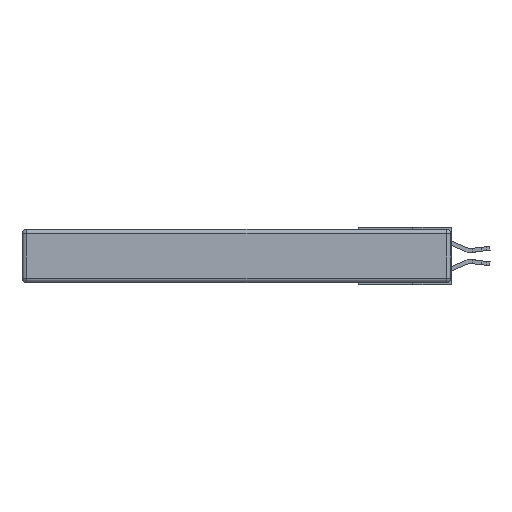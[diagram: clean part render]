
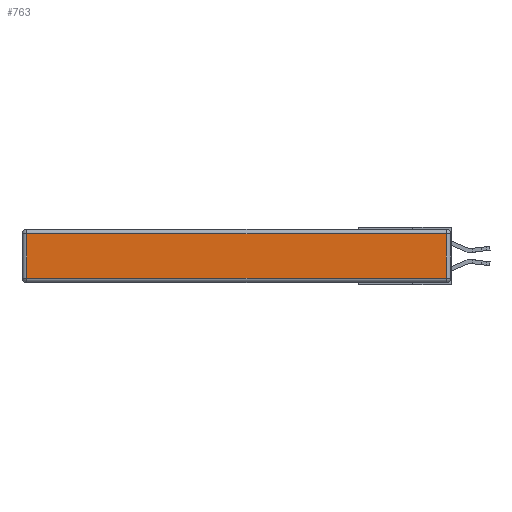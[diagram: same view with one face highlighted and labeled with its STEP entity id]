
A CAD part, left-side view. The second image highlights one B-rep face of the part: STEP entity #763.
In plain terms, the highlighted planar face has unit normal (-1, 0, 0).
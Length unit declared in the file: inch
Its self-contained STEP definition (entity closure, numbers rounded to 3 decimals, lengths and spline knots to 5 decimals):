
#692 = CARTESIAN_POINT ( 'NONE',  ( 0., 0., -0.343 ) ) ;
#763 = ADVANCED_FACE ( 'NONE', ( #19814 ), #5605, .T. ) ;
#936 = CARTESIAN_POINT ( 'NONE',  ( 0., 2.72, -0.313 ) ) ;
#1046 = CARTESIAN_POINT ( 'NONE',  ( 0., 0.03, -0.313 ) ) ;
#1474 = VECTOR ( 'NONE', #21287, 39.37008 ) ;
#1739 = LINE ( 'NONE', #4538, #1474 ) ;
#1753 = VECTOR ( 'NONE', #15206, 39.37008 ) ;
#2093 = EDGE_CURVE ( 'NONE', #3849, #6053, #13601, .T. ) ;
#2553 = EDGE_LOOP ( 'NONE', ( #14099, #6278, #18182, #12484 ) ) ;
#3849 = VERTEX_POINT ( 'NONE', #936 ) ;
#3950 = EDGE_CURVE ( 'NONE', #6053, #15411, #1739, .T. ) ;
#3998 = DIRECTION ( 'NONE',  ( 0., 0., 1. ) ) ;
#4538 = CARTESIAN_POINT ( 'NONE',  ( 0., 0.03, -0.343 ) ) ;
#5605 = PLANE ( 'NONE',  #11748 ) ;
#6053 = VERTEX_POINT ( 'NONE', #1046 ) ;
#6153 = CARTESIAN_POINT ( 'NONE',  ( 0., 0.03, -0.03 ) ) ;
#6278 = ORIENTED_EDGE ( 'NONE', *, *, #3950, .T. ) ;
#8877 = DIRECTION ( 'NONE',  ( -1., 0., 0. ) ) ;
#11748 = AXIS2_PLACEMENT_3D ( 'NONE', #692, #8877, #3998 ) ;
#12141 = VECTOR ( 'NONE', #12858, 39.37008 ) ;
#12484 = ORIENTED_EDGE ( 'NONE', *, *, #21196, .T. ) ;
#12858 = DIRECTION ( 'NONE',  ( 0., 0., -1. ) ) ;
#13451 = CARTESIAN_POINT ( 'NONE',  ( 0., 2.72, -0.343 ) ) ;
#13601 = LINE ( 'NONE', #14923, #16686 ) ;
#14099 = ORIENTED_EDGE ( 'NONE', *, *, #2093, .T. ) ;
#14923 = CARTESIAN_POINT ( 'NONE',  ( 0., 0., -0.313 ) ) ;
#14998 = LINE ( 'NONE', #16797, #1753 ) ;
#15101 = CARTESIAN_POINT ( 'NONE',  ( 0., 2.72, -0.03 ) ) ;
#15206 = DIRECTION ( 'NONE',  ( 0., 1., 0. ) ) ;
#15411 = VERTEX_POINT ( 'NONE', #6153 ) ;
#16686 = VECTOR ( 'NONE', #16854, 39.37008 ) ;
#16797 = CARTESIAN_POINT ( 'NONE',  ( 0., 2.75, -0.03 ) ) ;
#16854 = DIRECTION ( 'NONE',  ( 0., -1., 0. ) ) ;
#18081 = VERTEX_POINT ( 'NONE', #15101 ) ;
#18182 = ORIENTED_EDGE ( 'NONE', *, *, #20809, .T. ) ;
#19611 = LINE ( 'NONE', #13451, #12141 ) ;
#19814 = FACE_OUTER_BOUND ( 'NONE', #2553, .T. ) ;
#20809 = EDGE_CURVE ( 'NONE', #15411, #18081, #14998, .T. ) ;
#21196 = EDGE_CURVE ( 'NONE', #18081, #3849, #19611, .T. ) ;
#21287 = DIRECTION ( 'NONE',  ( 0., 0., 1. ) ) ;
